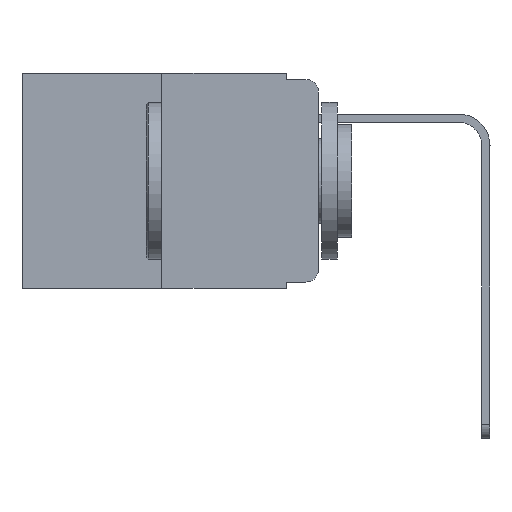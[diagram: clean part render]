
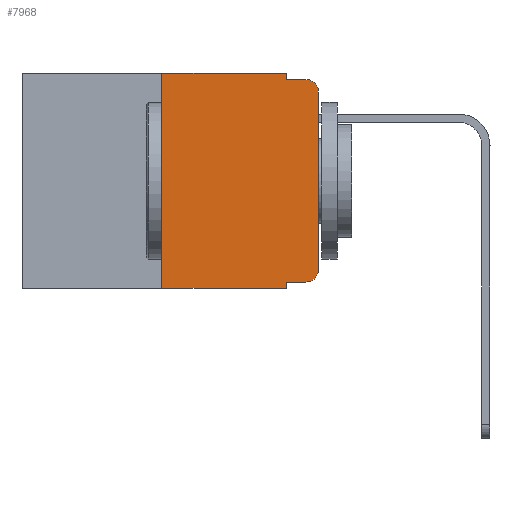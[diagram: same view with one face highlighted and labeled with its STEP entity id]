
A CAD part, left-side view. The second image highlights one B-rep face of the part: STEP entity #7968.
In plain terms, the highlighted planar face has unit normal (-1, 0, 0).
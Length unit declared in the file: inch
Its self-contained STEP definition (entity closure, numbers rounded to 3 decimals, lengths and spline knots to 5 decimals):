
#105 = CARTESIAN_POINT ( 'NONE',  ( 0., 0.051, -0.01 ) ) ;
#324 = ORIENTED_EDGE ( 'NONE', *, *, #10473, .F. ) ;
#514 = VERTEX_POINT ( 'NONE', #105 ) ;
#643 = LINE ( 'NONE', #16736, #17187 ) ;
#977 = DIRECTION ( 'NONE',  ( 0., -1., 0. ) ) ;
#1016 = EDGE_CURVE ( 'NONE', #1234, #15985, #11918, .T. ) ;
#1116 = PLANE ( 'NONE',  #7472 ) ;
#1188 = LINE ( 'NONE', #14951, #14983 ) ;
#1234 = VERTEX_POINT ( 'NONE', #15395 ) ;
#1596 = CARTESIAN_POINT ( 'NONE',  ( 0., 0.051, -0.333 ) ) ;
#1938 = LINE ( 'NONE', #9204, #8407 ) ;
#1949 = EDGE_CURVE ( 'NONE', #3023, #4203, #6224, .T. ) ;
#2274 = VECTOR ( 'NONE', #6601, 39.37008 ) ;
#2363 = DIRECTION ( 'NONE',  ( 0., -1., 0. ) ) ;
#2391 = EDGE_CURVE ( 'NONE', #15154, #13384, #1188, .T. ) ;
#2464 = DIRECTION ( 'NONE',  ( 1., 0., 0. ) ) ;
#2632 = EDGE_CURVE ( 'NONE', #514, #4203, #8710, .T. ) ;
#2727 = ORIENTED_EDGE ( 'NONE', *, *, #1016, .T. ) ;
#2808 = DIRECTION ( 'NONE',  ( 0., -1., 0. ) ) ;
#2988 = VERTEX_POINT ( 'NONE', #1596 ) ;
#3023 = VERTEX_POINT ( 'NONE', #8259 ) ;
#3697 = VECTOR ( 'NONE', #6398, 39.37008 ) ;
#3711 = CARTESIAN_POINT ( 'NONE',  ( 0., 0., 0. ) ) ;
#4203 = VERTEX_POINT ( 'NONE', #6845 ) ;
#4233 = VECTOR ( 'NONE', #15377, 39.37008 ) ;
#4294 = ORIENTED_EDGE ( 'NONE', *, *, #13134, .F. ) ;
#4589 = EDGE_CURVE ( 'NONE', #14112, #3023, #17325, .T. ) ;
#4796 = AXIS2_PLACEMENT_3D ( 'NONE', #11239, #13894, #8535 ) ;
#5771 = CARTESIAN_POINT ( 'NONE',  ( 0., 0.25, 0. ) ) ;
#6050 = DIRECTION ( 'NONE',  ( 0., 0., -1. ) ) ;
#6224 = CIRCLE ( 'NONE', #4796, 0.02 ) ;
#6398 = DIRECTION ( 'NONE',  ( 0., 0., 1. ) ) ;
#6601 = DIRECTION ( 'NONE',  ( 0., 0., -1. ) ) ;
#6834 = DIRECTION ( 'NONE',  ( -1., 0., 0. ) ) ;
#6845 = CARTESIAN_POINT ( 'NONE',  ( 0., 0.02, -0.01 ) ) ;
#7009 = DIRECTION ( 'NONE',  ( 0., -1., 0. ) ) ;
#7472 = AXIS2_PLACEMENT_3D ( 'NONE', #10486, #2464, #11834 ) ;
#7815 = AXIS2_PLACEMENT_3D ( 'NONE', #13535, #6834, #8177 ) ;
#7968 = ADVANCED_FACE ( 'NONE', ( #8803 ), #1116, .F. ) ;
#8177 = DIRECTION ( 'NONE',  ( 0., 0., -1. ) ) ;
#8259 = CARTESIAN_POINT ( 'NONE',  ( 0., 0., -0.03 ) ) ;
#8407 = VECTOR ( 'NONE', #977, 39.37008 ) ;
#8492 = ORIENTED_EDGE ( 'NONE', *, *, #9063, .F. ) ;
#8535 = DIRECTION ( 'NONE',  ( 0., 0., -1. ) ) ;
#8710 = LINE ( 'NONE', #11044, #13540 ) ;
#8803 = FACE_OUTER_BOUND ( 'NONE', #13703, .T. ) ;
#9063 = EDGE_CURVE ( 'NONE', #2988, #15985, #643, .T. ) ;
#9204 = CARTESIAN_POINT ( 'NONE',  ( 0., 0.051, -0.333 ) ) ;
#9459 = EDGE_CURVE ( 'NONE', #9892, #14112, #12982, .T. ) ;
#9789 = ORIENTED_EDGE ( 'NONE', *, *, #2632, .F. ) ;
#9892 = VERTEX_POINT ( 'NONE', #16880 ) ;
#9921 = LINE ( 'NONE', #5771, #4233 ) ;
#10398 = CARTESIAN_POINT ( 'NONE',  ( 0., 0.473, -0.343 ) ) ;
#10473 = EDGE_CURVE ( 'NONE', #1234, #15154, #9921, .T. ) ;
#10486 = CARTESIAN_POINT ( 'NONE',  ( 0., 0.473, 0. ) ) ;
#10765 = CARTESIAN_POINT ( 'NONE',  ( 0., 0., -0.313 ) ) ;
#11044 = CARTESIAN_POINT ( 'NONE',  ( 0., 0.051, -0.01 ) ) ;
#11239 = CARTESIAN_POINT ( 'NONE',  ( 0., 0.02, -0.03 ) ) ;
#11710 = ORIENTED_EDGE ( 'NONE', *, *, #9459, .T. ) ;
#11834 = DIRECTION ( 'NONE',  ( 0., 0., -1. ) ) ;
#11918 = LINE ( 'NONE', #10398, #12784 ) ;
#12168 = ORIENTED_EDGE ( 'NONE', *, *, #4589, .T. ) ;
#12228 = ORIENTED_EDGE ( 'NONE', *, *, #12619, .T. ) ;
#12352 = CARTESIAN_POINT ( 'NONE',  ( 0., 0.051, -0.343 ) ) ;
#12619 = EDGE_CURVE ( 'NONE', #2988, #9892, #1938, .T. ) ;
#12759 = LINE ( 'NONE', #15906, #2274 ) ;
#12784 = VECTOR ( 'NONE', #2363, 39.37008 ) ;
#12982 = CIRCLE ( 'NONE', #7815, 0.02 ) ;
#13134 = EDGE_CURVE ( 'NONE', #13384, #514, #12759, .T. ) ;
#13384 = VERTEX_POINT ( 'NONE', #16923 ) ;
#13535 = CARTESIAN_POINT ( 'NONE',  ( 0., 0.02, -0.313 ) ) ;
#13540 = VECTOR ( 'NONE', #7009, 39.37008 ) ;
#13703 = EDGE_LOOP ( 'NONE', ( #12168, #17287, #9789, #4294, #16229, #324, #2727, #8492, #12228, #11710 ) ) ;
#13894 = DIRECTION ( 'NONE',  ( -1., 0., 0. ) ) ;
#14112 = VERTEX_POINT ( 'NONE', #10765 ) ;
#14951 = CARTESIAN_POINT ( 'NONE',  ( 0., 0.473, 0. ) ) ;
#14983 = VECTOR ( 'NONE', #2808, 39.37008 ) ;
#15154 = VERTEX_POINT ( 'NONE', #16011 ) ;
#15377 = DIRECTION ( 'NONE',  ( 0., 0., 1. ) ) ;
#15395 = CARTESIAN_POINT ( 'NONE',  ( 0., 0.25, -0.343 ) ) ;
#15906 = CARTESIAN_POINT ( 'NONE',  ( 0., 0.051, 0. ) ) ;
#15985 = VERTEX_POINT ( 'NONE', #12352 ) ;
#16011 = CARTESIAN_POINT ( 'NONE',  ( 0., 0.25, 0. ) ) ;
#16229 = ORIENTED_EDGE ( 'NONE', *, *, #2391, .F. ) ;
#16736 = CARTESIAN_POINT ( 'NONE',  ( 0., 0.051, 0. ) ) ;
#16880 = CARTESIAN_POINT ( 'NONE',  ( 0., 0.02, -0.333 ) ) ;
#16923 = CARTESIAN_POINT ( 'NONE',  ( 0., 0.051, 0. ) ) ;
#17187 = VECTOR ( 'NONE', #6050, 39.37008 ) ;
#17287 = ORIENTED_EDGE ( 'NONE', *, *, #1949, .T. ) ;
#17325 = LINE ( 'NONE', #3711, #3697 ) ;
